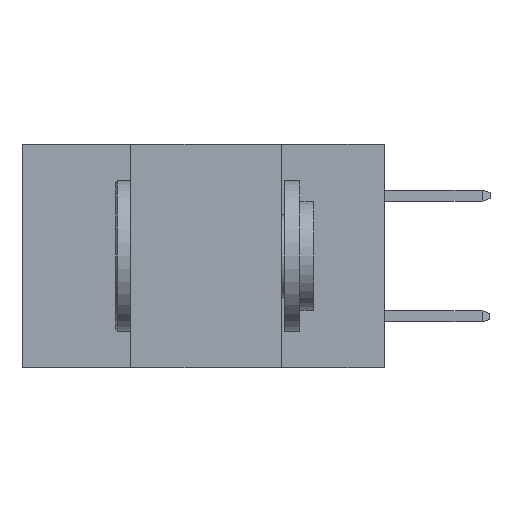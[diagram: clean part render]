
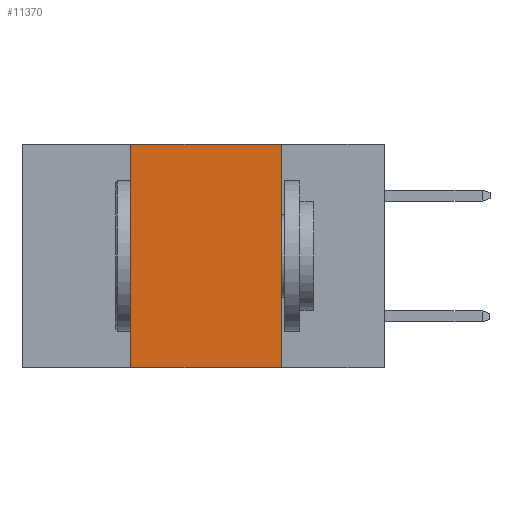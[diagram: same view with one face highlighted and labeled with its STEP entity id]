
A CAD part, left-side view. The second image highlights one B-rep face of the part: STEP entity #11370.
In plain terms, the highlighted planar face has unit normal (-1, 0, 0).
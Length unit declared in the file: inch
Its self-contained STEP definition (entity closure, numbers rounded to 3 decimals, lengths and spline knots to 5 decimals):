
#518 = EDGE_CURVE ( 'NONE', #4367, #5393, #14845, .T. ) ;
#1000 = VECTOR ( 'NONE', #9108, 39.37008 ) ;
#1465 = CARTESIAN_POINT ( 'NONE',  ( 0., 0.42, 0. ) ) ;
#2781 = ORIENTED_EDGE ( 'NONE', *, *, #518, .T. ) ;
#2806 = EDGE_CURVE ( 'NONE', #8706, #5393, #4673, .T. ) ;
#4367 = VERTEX_POINT ( 'NONE', #9697 ) ;
#4553 = EDGE_LOOP ( 'NONE', ( #6383, #7990, #9133, #2781 ) ) ;
#4624 = CARTESIAN_POINT ( 'NONE',  ( 0., 0.6, 0. ) ) ;
#4673 = LINE ( 'NONE', #10431, #1000 ) ;
#4735 = VECTOR ( 'NONE', #9687, 39.37008 ) ;
#4829 = FACE_OUTER_BOUND ( 'NONE', #4553, .T. ) ;
#5393 = VERTEX_POINT ( 'NONE', #14405 ) ;
#5625 = DIRECTION ( 'NONE',  ( 0., 0., 1. ) ) ;
#5791 = DIRECTION ( 'NONE',  ( 1., 0., 0. ) ) ;
#6086 = CARTESIAN_POINT ( 'NONE',  ( 0., 0.6, 0. ) ) ;
#6383 = ORIENTED_EDGE ( 'NONE', *, *, #2806, .F. ) ;
#6734 = CARTESIAN_POINT ( 'NONE',  ( 0., 0.42, 0. ) ) ;
#7863 = LINE ( 'NONE', #6086, #4735 ) ;
#7990 = ORIENTED_EDGE ( 'NONE', *, *, #13986, .F. ) ;
#8526 = VECTOR ( 'NONE', #5625, 39.37008 ) ;
#8706 = VERTEX_POINT ( 'NONE', #13173 ) ;
#9108 = DIRECTION ( 'NONE',  ( 0., 0., -1. ) ) ;
#9133 = ORIENTED_EDGE ( 'NONE', *, *, #11944, .F. ) ;
#9687 = DIRECTION ( 'NONE',  ( 0., -1., 0. ) ) ;
#9697 = CARTESIAN_POINT ( 'NONE',  ( 0., 0.42, -0.37 ) ) ;
#10275 = DIRECTION ( 'NONE',  ( 0., -1., 0. ) ) ;
#10431 = CARTESIAN_POINT ( 'NONE',  ( 0., 0.17, 0. ) ) ;
#11370 = ADVANCED_FACE ( 'NONE', ( #4829 ), #11672, .F. ) ;
#11623 = LINE ( 'NONE', #6734, #8526 ) ;
#11672 = PLANE ( 'NONE',  #14673 ) ;
#11944 = EDGE_CURVE ( 'NONE', #4367, #15285, #11623, .T. ) ;
#13173 = CARTESIAN_POINT ( 'NONE',  ( 0., 0.17, 0. ) ) ;
#13551 = CARTESIAN_POINT ( 'NONE',  ( 0., 0.6, -0.37 ) ) ;
#13986 = EDGE_CURVE ( 'NONE', #15285, #8706, #7863, .T. ) ;
#13988 = DIRECTION ( 'NONE',  ( 0., 0., -1. ) ) ;
#14405 = CARTESIAN_POINT ( 'NONE',  ( 0., 0.17, -0.37 ) ) ;
#14502 = VECTOR ( 'NONE', #10275, 39.37008 ) ;
#14673 = AXIS2_PLACEMENT_3D ( 'NONE', #4624, #5791, #13988 ) ;
#14845 = LINE ( 'NONE', #13551, #14502 ) ;
#15285 = VERTEX_POINT ( 'NONE', #1465 ) ;
